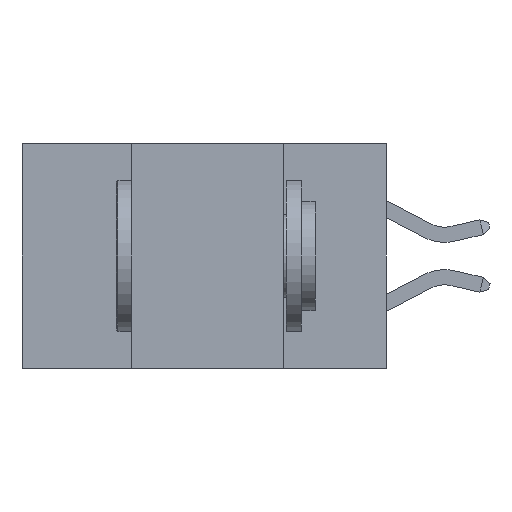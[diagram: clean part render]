
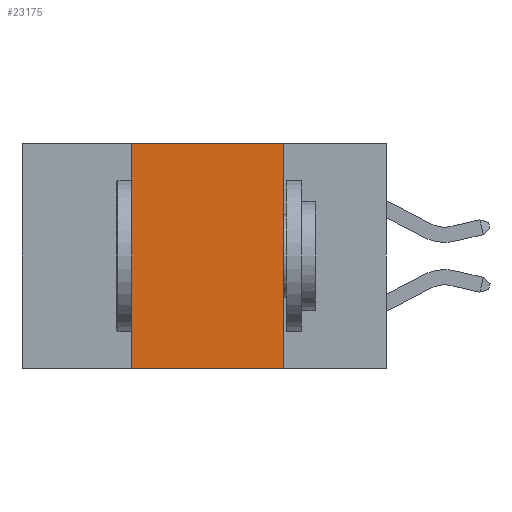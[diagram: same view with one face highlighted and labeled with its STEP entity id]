
A CAD part, left-side view. The second image highlights one B-rep face of the part: STEP entity #23175.
In plain terms, the highlighted planar face has unit normal (-1, 0, 0).
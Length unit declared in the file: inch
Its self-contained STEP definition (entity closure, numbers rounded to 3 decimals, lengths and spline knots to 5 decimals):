
#1568 = VERTEX_POINT ( 'NONE', #3286 ) ;
#2062 = EDGE_LOOP ( 'NONE', ( #19673, #14294, #13148, #2678 ) ) ;
#2678 = ORIENTED_EDGE ( 'NONE', *, *, #6326, .T. ) ;
#3286 = CARTESIAN_POINT ( 'NONE',  ( 0., 0.17, 0. ) ) ;
#3870 = VECTOR ( 'NONE', #8191, 39.37008 ) ;
#4290 = CARTESIAN_POINT ( 'NONE',  ( 0., 0.42, -0.37 ) ) ;
#5255 = CARTESIAN_POINT ( 'NONE',  ( 0., 0.17, -0.37 ) ) ;
#5256 = DIRECTION ( 'NONE',  ( 0., 0., 1. ) ) ;
#6326 = EDGE_CURVE ( 'NONE', #14241, #19100, #15162, .T. ) ;
#7444 = VECTOR ( 'NONE', #19187, 39.37008 ) ;
#8191 = DIRECTION ( 'NONE',  ( 0., -1., 0. ) ) ;
#8671 = EDGE_CURVE ( 'NONE', #14241, #23128, #16254, .T. ) ;
#9460 = CARTESIAN_POINT ( 'NONE',  ( 0., 0.6, -0.37 ) ) ;
#10661 = AXIS2_PLACEMENT_3D ( 'NONE', #10899, #23796, #12797 ) ;
#10899 = CARTESIAN_POINT ( 'NONE',  ( 0., 0.6, 0. ) ) ;
#12797 = DIRECTION ( 'NONE',  ( 0., 0., -1. ) ) ;
#13148 = ORIENTED_EDGE ( 'NONE', *, *, #8671, .F. ) ;
#13155 = LINE ( 'NONE', #17349, #7444 ) ;
#13525 = LINE ( 'NONE', #21254, #3870 ) ;
#14241 = VERTEX_POINT ( 'NONE', #4290 ) ;
#14294 = ORIENTED_EDGE ( 'NONE', *, *, #18083, .F. ) ;
#14451 = CARTESIAN_POINT ( 'NONE',  ( 0., 0.42, 0. ) ) ;
#15162 = LINE ( 'NONE', #9460, #20010 ) ;
#15689 = VECTOR ( 'NONE', #5256, 39.37008 ) ;
#16254 = LINE ( 'NONE', #18542, #15689 ) ;
#17349 = CARTESIAN_POINT ( 'NONE',  ( 0., 0.17, -0.37 ) ) ;
#18083 = EDGE_CURVE ( 'NONE', #23128, #1568, #13525, .T. ) ;
#18542 = CARTESIAN_POINT ( 'NONE',  ( 0., 0.42, -0.37 ) ) ;
#19100 = VERTEX_POINT ( 'NONE', #5255 ) ;
#19187 = DIRECTION ( 'NONE',  ( 0., 0., -1. ) ) ;
#19673 = ORIENTED_EDGE ( 'NONE', *, *, #23915, .F. ) ;
#20010 = VECTOR ( 'NONE', #22434, 39.37008 ) ;
#20112 = FACE_OUTER_BOUND ( 'NONE', #2062, .T. ) ;
#21254 = CARTESIAN_POINT ( 'NONE',  ( 0., 0.6, 0. ) ) ;
#21985 = PLANE ( 'NONE',  #10661 ) ;
#22434 = DIRECTION ( 'NONE',  ( 0., -1., 0. ) ) ;
#23128 = VERTEX_POINT ( 'NONE', #14451 ) ;
#23175 = ADVANCED_FACE ( 'NONE', ( #20112 ), #21985, .F. ) ;
#23796 = DIRECTION ( 'NONE',  ( 1., 0., 0. ) ) ;
#23915 = EDGE_CURVE ( 'NONE', #1568, #19100, #13155, .T. ) ;
